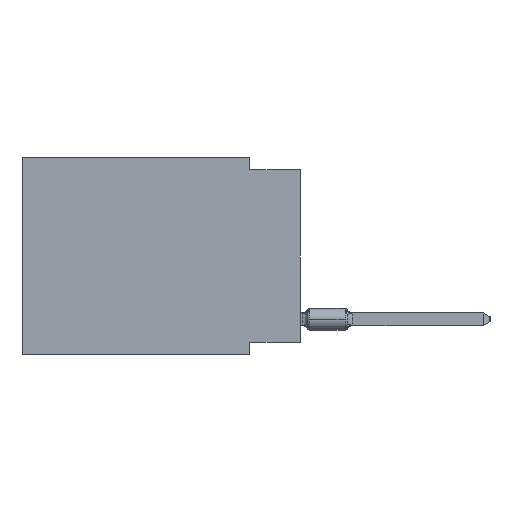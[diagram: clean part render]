
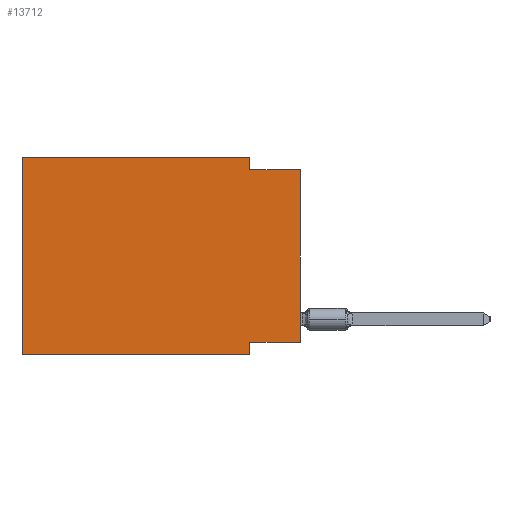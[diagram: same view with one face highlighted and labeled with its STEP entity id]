
A CAD part, left-side view. The second image highlights one B-rep face of the part: STEP entity #13712.
In plain terms, the highlighted planar face has unit normal (-1, 0, 0).
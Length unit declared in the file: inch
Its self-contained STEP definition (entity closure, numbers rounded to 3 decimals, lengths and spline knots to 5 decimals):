
#184 = PLANE ( 'NONE',  #19841 ) ;
#826 = LINE ( 'NONE', #3705, #24245 ) ;
#841 = EDGE_CURVE ( 'NONE', #23798, #10776, #826, .T. ) ;
#1337 = DIRECTION ( 'NONE',  ( 0., 1., 0. ) ) ;
#1545 = VERTEX_POINT ( 'NONE', #14158 ) ;
#2604 = VECTOR ( 'NONE', #14220, 39.37008 ) ;
#2933 = LINE ( 'NONE', #10862, #23918 ) ;
#3503 = CARTESIAN_POINT ( 'NONE',  ( 0., 0.1, -0.025 ) ) ;
#3660 = ORIENTED_EDGE ( 'NONE', *, *, #15831, .T. ) ;
#3705 = CARTESIAN_POINT ( 'NONE',  ( 0., 0.55, 0. ) ) ;
#3842 = CARTESIAN_POINT ( 'NONE',  ( 0., 0.55, 0. ) ) ;
#6399 = DIRECTION ( 'NONE',  ( 0., -1., 0. ) ) ;
#6498 = CARTESIAN_POINT ( 'NONE',  ( 0., 0., -0.025 ) ) ;
#7362 = DIRECTION ( 'NONE',  ( 0., 0., -1. ) ) ;
#7829 = LINE ( 'NONE', #31279, #18185 ) ;
#8213 = VECTOR ( 'NONE', #7362, 39.37008 ) ;
#8737 = CARTESIAN_POINT ( 'NONE',  ( 0., 0.1, 0. ) ) ;
#8746 = VECTOR ( 'NONE', #1337, 39.37008 ) ;
#9810 = EDGE_CURVE ( 'NONE', #27438, #23798, #19689, .T. ) ;
#10699 = DIRECTION ( 'NONE',  ( 0., 0., -1. ) ) ;
#10776 = VERTEX_POINT ( 'NONE', #8737 ) ;
#10862 = CARTESIAN_POINT ( 'NONE',  ( 0., 0.55, -0.39 ) ) ;
#11161 = CARTESIAN_POINT ( 'NONE',  ( 0., 0.55, -0.39 ) ) ;
#11410 = VERTEX_POINT ( 'NONE', #27570 ) ;
#12835 = EDGE_CURVE ( 'NONE', #15855, #1545, #7829, .T. ) ;
#13222 = ORIENTED_EDGE ( 'NONE', *, *, #841, .F. ) ;
#13228 = DIRECTION ( 'NONE',  ( 0., -1., 0. ) ) ;
#13712 = ADVANCED_FACE ( 'NONE', ( #19193 ), #184, .F. ) ;
#14112 = ORIENTED_EDGE ( 'NONE', *, *, #9810, .F. ) ;
#14128 = DIRECTION ( 'NONE',  ( 0., 0., 1. ) ) ;
#14158 = CARTESIAN_POINT ( 'NONE',  ( 0., 0.1, -0.39 ) ) ;
#14220 = DIRECTION ( 'NONE',  ( 0., 0., 1. ) ) ;
#14319 = EDGE_CURVE ( 'NONE', #18409, #30592, #14413, .T. ) ;
#14413 = LINE ( 'NONE', #6498, #18260 ) ;
#15831 = EDGE_CURVE ( 'NONE', #11410, #30592, #24513, .T. ) ;
#15855 = VERTEX_POINT ( 'NONE', #24681 ) ;
#16955 = ORIENTED_EDGE ( 'NONE', *, *, #12835, .F. ) ;
#18185 = VECTOR ( 'NONE', #10699, 39.37008 ) ;
#18260 = VECTOR ( 'NONE', #27084, 39.37008 ) ;
#18409 = VERTEX_POINT ( 'NONE', #3503 ) ;
#18687 = CARTESIAN_POINT ( 'NONE',  ( 0., 0.55, 0. ) ) ;
#19193 = FACE_OUTER_BOUND ( 'NONE', #21652, .T. ) ;
#19685 = CARTESIAN_POINT ( 'NONE',  ( 0., 0., -0.025 ) ) ;
#19689 = LINE ( 'NONE', #3842, #32722 ) ;
#19841 = AXIS2_PLACEMENT_3D ( 'NONE', #18687, #23135, #31835 ) ;
#19872 = ORIENTED_EDGE ( 'NONE', *, *, #14319, .F. ) ;
#21011 = ORIENTED_EDGE ( 'NONE', *, *, #24531, .T. ) ;
#21652 = EDGE_LOOP ( 'NONE', ( #3660, #19872, #32041, #13222, #14112, #21011, #16955, #28402 ) ) ;
#21759 = LINE ( 'NONE', #29519, #8746 ) ;
#23135 = DIRECTION ( 'NONE',  ( 1., 0., 0. ) ) ;
#23223 = CARTESIAN_POINT ( 'NONE',  ( 0., 0.1, 0. ) ) ;
#23798 = VERTEX_POINT ( 'NONE', #33154 ) ;
#23918 = VECTOR ( 'NONE', #13228, 39.37008 ) ;
#24245 = VECTOR ( 'NONE', #6399, 39.37008 ) ;
#24513 = LINE ( 'NONE', #29412, #2604 ) ;
#24531 = EDGE_CURVE ( 'NONE', #27438, #1545, #2933, .T. ) ;
#24681 = CARTESIAN_POINT ( 'NONE',  ( 0., 0.1, -0.365 ) ) ;
#25250 = LINE ( 'NONE', #23223, #8213 ) ;
#27084 = DIRECTION ( 'NONE',  ( 0., -1., 0. ) ) ;
#27438 = VERTEX_POINT ( 'NONE', #11161 ) ;
#27570 = CARTESIAN_POINT ( 'NONE',  ( 0., 0., -0.365 ) ) ;
#28402 = ORIENTED_EDGE ( 'NONE', *, *, #30146, .F. ) ;
#29412 = CARTESIAN_POINT ( 'NONE',  ( 0., 0., 0. ) ) ;
#29519 = CARTESIAN_POINT ( 'NONE',  ( 0., 0., -0.365 ) ) ;
#30146 = EDGE_CURVE ( 'NONE', #11410, #15855, #21759, .T. ) ;
#30592 = VERTEX_POINT ( 'NONE', #19685 ) ;
#31279 = CARTESIAN_POINT ( 'NONE',  ( 0., 0.1, -0.39 ) ) ;
#31835 = DIRECTION ( 'NONE',  ( 0., 0., -1. ) ) ;
#31945 = EDGE_CURVE ( 'NONE', #10776, #18409, #25250, .T. ) ;
#32041 = ORIENTED_EDGE ( 'NONE', *, *, #31945, .F. ) ;
#32722 = VECTOR ( 'NONE', #14128, 39.37008 ) ;
#33154 = CARTESIAN_POINT ( 'NONE',  ( 0., 0.55, 0. ) ) ;
